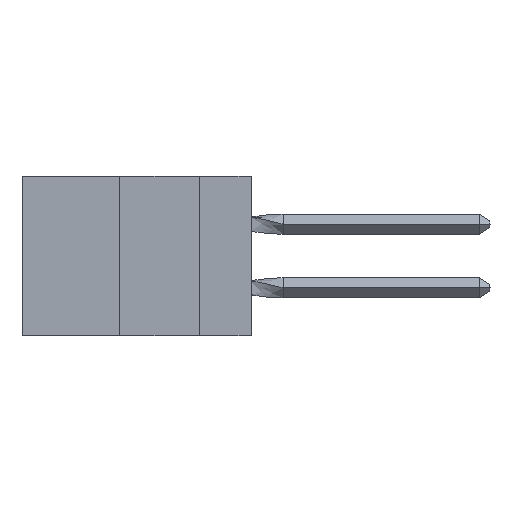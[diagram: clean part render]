
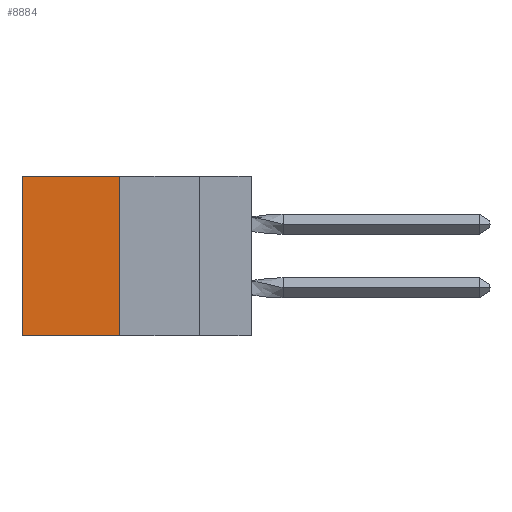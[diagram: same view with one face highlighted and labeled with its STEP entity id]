
A CAD part, left-side view. The second image highlights one B-rep face of the part: STEP entity #8884.
In plain terms, the highlighted planar face has unit normal (-1, 0, 0).
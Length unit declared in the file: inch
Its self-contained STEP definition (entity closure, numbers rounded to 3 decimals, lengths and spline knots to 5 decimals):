
#682 = PLANE ( 'NONE',  #9281 ) ;
#804 = DIRECTION ( 'NONE',  ( 0., 0., -1. ) ) ;
#2077 = EDGE_CURVE ( 'NONE', #4195, #8907, #14167, .T. ) ;
#2150 = CARTESIAN_POINT ( 'NONE',  ( 0.305, 0.72, -0.5 ) ) ;
#2689 = ORIENTED_EDGE ( 'NONE', *, *, #7689, .T. ) ;
#2873 = EDGE_LOOP ( 'NONE', ( #3968, #13241, #3226, #2689 ) ) ;
#3067 = CARTESIAN_POINT ( 'NONE',  ( 0.305, 0.72, -0.5 ) ) ;
#3226 = ORIENTED_EDGE ( 'NONE', *, *, #6351, .F. ) ;
#3931 = CARTESIAN_POINT ( 'NONE',  ( 0.305, 0.413, -0.5 ) ) ;
#3968 = ORIENTED_EDGE ( 'NONE', *, *, #6355, .T. ) ;
#4195 = VERTEX_POINT ( 'NONE', #7819 ) ;
#5566 = DIRECTION ( 'NONE',  ( 0., 1., 0. ) ) ;
#5888 = CARTESIAN_POINT ( 'NONE',  ( 0.305, 0.413, -0.5 ) ) ;
#6351 = EDGE_CURVE ( 'NONE', #7558, #4195, #16164, .T. ) ;
#6355 = EDGE_CURVE ( 'NONE', #15202, #8907, #15780, .T. ) ;
#6850 = DIRECTION ( 'NONE',  ( 0., 0., -1. ) ) ;
#7317 = FACE_OUTER_BOUND ( 'NONE', #2873, .T. ) ;
#7558 = VERTEX_POINT ( 'NONE', #14287 ) ;
#7588 = DIRECTION ( 'NONE',  ( 0., 1., 0. ) ) ;
#7689 = EDGE_CURVE ( 'NONE', #7558, #15202, #12649, .T. ) ;
#7819 = CARTESIAN_POINT ( 'NONE',  ( 0.305, 0.413, -0.5 ) ) ;
#8880 = VECTOR ( 'NONE', #5566, 39.37008 ) ;
#8884 = ADVANCED_FACE ( 'NONE', ( #7317 ), #682, .F. ) ;
#8907 = VERTEX_POINT ( 'NONE', #3067 ) ;
#9281 = AXIS2_PLACEMENT_3D ( 'NONE', #9610, #14447, #6850 ) ;
#9610 = CARTESIAN_POINT ( 'NONE',  ( 0.305, 0.413, -0.5 ) ) ;
#11301 = CARTESIAN_POINT ( 'NONE',  ( 0.305, 0.72, 0. ) ) ;
#12021 = CARTESIAN_POINT ( 'NONE',  ( 0.305, 0.413, 0. ) ) ;
#12377 = VECTOR ( 'NONE', #14878, 39.37008 ) ;
#12388 = VECTOR ( 'NONE', #7588, 39.37008 ) ;
#12649 = LINE ( 'NONE', #12021, #8880 ) ;
#12784 = VECTOR ( 'NONE', #804, 39.37008 ) ;
#13241 = ORIENTED_EDGE ( 'NONE', *, *, #2077, .F. ) ;
#14167 = LINE ( 'NONE', #3931, #12388 ) ;
#14287 = CARTESIAN_POINT ( 'NONE',  ( 0.305, 0.413, 0. ) ) ;
#14447 = DIRECTION ( 'NONE',  ( 1., 0., 0. ) ) ;
#14878 = DIRECTION ( 'NONE',  ( 0., 0., -1. ) ) ;
#15202 = VERTEX_POINT ( 'NONE', #11301 ) ;
#15780 = LINE ( 'NONE', #2150, #12377 ) ;
#16164 = LINE ( 'NONE', #5888, #12784 ) ;
